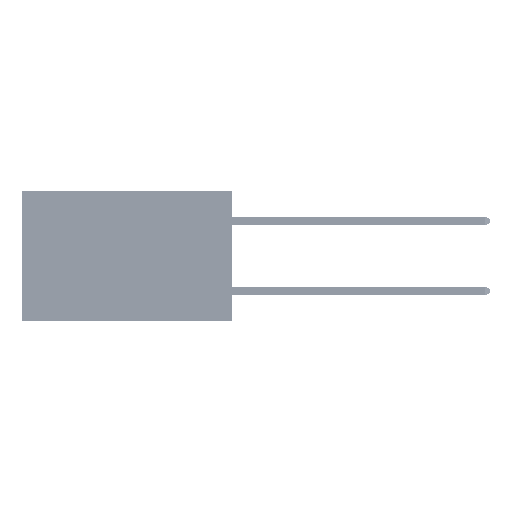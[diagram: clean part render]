
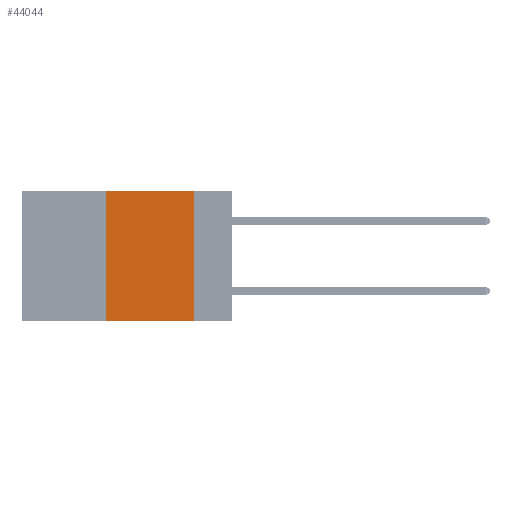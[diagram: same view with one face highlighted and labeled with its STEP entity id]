
A CAD part, left-side view. The second image highlights one B-rep face of the part: STEP entity #44044.
In plain terms, the highlighted planar face has unit normal (-1, 0, 0).
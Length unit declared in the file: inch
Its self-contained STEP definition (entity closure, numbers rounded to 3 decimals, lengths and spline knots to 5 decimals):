
#785 = EDGE_CURVE ( 'NONE', #18926, #4092, #50097, .T. ) ;
#1057 = ORIENTED_EDGE ( 'NONE', *, *, #7687, .F. ) ;
#1802 = CARTESIAN_POINT ( 'NONE',  ( 0., 0.6, -0.37 ) ) ;
#4092 = VERTEX_POINT ( 'NONE', #19426 ) ;
#7386 = LINE ( 'NONE', #19043, #10669 ) ;
#7687 = EDGE_CURVE ( 'NONE', #7738, #16496, #7386, .T. ) ;
#7738 = VERTEX_POINT ( 'NONE', #27041 ) ;
#10116 = DIRECTION ( 'NONE',  ( 0., 0., 1. ) ) ;
#10207 = LINE ( 'NONE', #10460, #45917 ) ;
#10374 = LINE ( 'NONE', #14610, #48378 ) ;
#10460 = CARTESIAN_POINT ( 'NONE',  ( 0., 0.11, 0. ) ) ;
#10669 = VECTOR ( 'NONE', #43236, 39.37008 ) ;
#12901 = EDGE_CURVE ( 'NONE', #16496, #4092, #10207, .T. ) ;
#14610 = CARTESIAN_POINT ( 'NONE',  ( 0., 0.36, 0. ) ) ;
#15336 = AXIS2_PLACEMENT_3D ( 'NONE', #51381, #47423, #50603 ) ;
#15593 = ORIENTED_EDGE ( 'NONE', *, *, #12901, .F. ) ;
#16496 = VERTEX_POINT ( 'NONE', #18824 ) ;
#17970 = CARTESIAN_POINT ( 'NONE',  ( 0., 0.36, -0.37 ) ) ;
#18214 = FACE_OUTER_BOUND ( 'NONE', #41878, .T. ) ;
#18824 = CARTESIAN_POINT ( 'NONE',  ( 0., 0.11, 0. ) ) ;
#18926 = VERTEX_POINT ( 'NONE', #17970 ) ;
#19043 = CARTESIAN_POINT ( 'NONE',  ( 0., 0.6, 0. ) ) ;
#19426 = CARTESIAN_POINT ( 'NONE',  ( 0., 0.11, -0.37 ) ) ;
#21960 = DIRECTION ( 'NONE',  ( 0., -1., 0. ) ) ;
#26291 = EDGE_CURVE ( 'NONE', #18926, #7738, #10374, .T. ) ;
#26728 = PLANE ( 'NONE',  #15336 ) ;
#27041 = CARTESIAN_POINT ( 'NONE',  ( 0., 0.36, 0. ) ) ;
#36648 = ORIENTED_EDGE ( 'NONE', *, *, #785, .T. ) ;
#37954 = VECTOR ( 'NONE', #21960, 39.37008 ) ;
#39462 = ORIENTED_EDGE ( 'NONE', *, *, #26291, .F. ) ;
#41878 = EDGE_LOOP ( 'NONE', ( #15593, #1057, #39462, #36648 ) ) ;
#43236 = DIRECTION ( 'NONE',  ( 0., -1., 0. ) ) ;
#44044 = ADVANCED_FACE ( 'NONE', ( #18214 ), #26728, .F. ) ;
#45917 = VECTOR ( 'NONE', #46305, 39.37008 ) ;
#46305 = DIRECTION ( 'NONE',  ( 0., 0., -1. ) ) ;
#47423 = DIRECTION ( 'NONE',  ( 1., 0., 0. ) ) ;
#48378 = VECTOR ( 'NONE', #10116, 39.37008 ) ;
#50097 = LINE ( 'NONE', #1802, #37954 ) ;
#50603 = DIRECTION ( 'NONE',  ( 0., 0., -1. ) ) ;
#51381 = CARTESIAN_POINT ( 'NONE',  ( 0., 0.6, 0. ) ) ;
